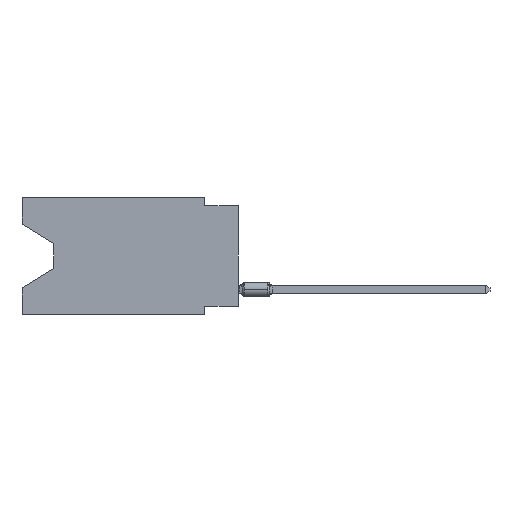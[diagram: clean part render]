
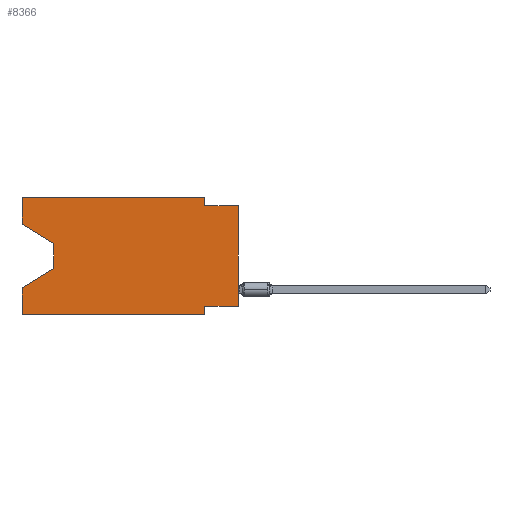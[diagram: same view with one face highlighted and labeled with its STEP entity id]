
A CAD part, left-side view. The second image highlights one B-rep face of the part: STEP entity #8366.
In plain terms, the highlighted planar face has unit normal (-1, 0, 0).
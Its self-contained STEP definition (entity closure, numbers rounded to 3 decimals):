
#251 = LINE ( 'NONE', #2073, #12682 ) ;
#1087 = VERTEX_POINT ( 'NONE', #7976 ) ;
#1093 = LINE ( 'NONE', #2813, #13261 ) ;
#1193 = DIRECTION ( 'NONE',  ( 0., -0.855, -0.519 ) ) ;
#1688 = LINE ( 'NONE', #13062, #12560 ) ;
#1826 = CARTESIAN_POINT ( 'NONE',  ( 0., 0., -0.635 ) ) ;
#1995 = EDGE_CURVE ( 'NONE', #4940, #10444, #19804, .T. ) ;
#2073 = CARTESIAN_POINT ( 'NONE',  ( 0., 16.383, 0. ) ) ;
#2531 = CARTESIAN_POINT ( 'NONE',  ( 0., 0., 0. ) ) ;
#2554 = EDGE_CURVE ( 'NONE', #6788, #12867, #10756, .T. ) ;
#2598 = CARTESIAN_POINT ( 'NONE',  ( 0., 16.383, -2.038 ) ) ;
#2666 = EDGE_CURVE ( 'NONE', #1087, #6656, #3111, .T. ) ;
#2712 = CARTESIAN_POINT ( 'NONE',  ( 0., 2.54, -0.635 ) ) ;
#2813 = CARTESIAN_POINT ( 'NONE',  ( 0., 16.383, 0. ) ) ;
#2944 = DIRECTION ( 'NONE',  ( 0., 0., -1. ) ) ;
#3111 = LINE ( 'NONE', #9673, #4296 ) ;
#3185 = CARTESIAN_POINT ( 'NONE',  ( 0., 16.383, -6.852 ) ) ;
#3435 = VECTOR ( 'NONE', #15576, 1000. ) ;
#3577 = ORIENTED_EDGE ( 'NONE', *, *, #8878, .F. ) ;
#4155 = LINE ( 'NONE', #7382, #7997 ) ;
#4232 = VECTOR ( 'NONE', #18378, 1000. ) ;
#4296 = VECTOR ( 'NONE', #14611, 1000. ) ;
#4940 = VERTEX_POINT ( 'NONE', #19956 ) ;
#5105 = ORIENTED_EDGE ( 'NONE', *, *, #1995, .T. ) ;
#5122 = CARTESIAN_POINT ( 'NONE',  ( 0., 16.383, -8.89 ) ) ;
#5468 = AXIS2_PLACEMENT_3D ( 'NONE', #16095, #17806, #19206 ) ;
#5704 = CARTESIAN_POINT ( 'NONE',  ( 0., 0., -0.635 ) ) ;
#6019 = FACE_OUTER_BOUND ( 'NONE', #6033, .T. ) ;
#6023 = LINE ( 'NONE', #5704, #3435 ) ;
#6033 = EDGE_LOOP ( 'NONE', ( #15017, #9505, #20596, #15298, #5105, #17332, #7921, #18885, #9639, #10597, #13761, #3577 ) ) ;
#6114 = LINE ( 'NONE', #9434, #14827 ) ;
#6656 = VERTEX_POINT ( 'NONE', #3185 ) ;
#6788 = VERTEX_POINT ( 'NONE', #15306 ) ;
#7232 = DIRECTION ( 'NONE',  ( 0., 0., 1. ) ) ;
#7358 = VERTEX_POINT ( 'NONE', #12612 ) ;
#7382 = CARTESIAN_POINT ( 'NONE',  ( 0., 13.97, -3.505 ) ) ;
#7545 = VECTOR ( 'NONE', #18416, 1000. ) ;
#7596 = EDGE_CURVE ( 'NONE', #7358, #9245, #8733, .T. ) ;
#7603 = VECTOR ( 'NONE', #2944, 1000. ) ;
#7921 = ORIENTED_EDGE ( 'NONE', *, *, #7596, .F. ) ;
#7976 = CARTESIAN_POINT ( 'NONE',  ( 0., 13.97, -5.385 ) ) ;
#7997 = VECTOR ( 'NONE', #10701, 1000. ) ;
#8366 = ADVANCED_FACE ( 'NONE', ( #6019 ), #10959, .F. ) ;
#8733 = LINE ( 'NONE', #13456, #4232 ) ;
#8878 = EDGE_CURVE ( 'NONE', #6788, #16752, #251, .T. ) ;
#9245 = VERTEX_POINT ( 'NONE', #19967 ) ;
#9284 = LINE ( 'NONE', #14424, #7603 ) ;
#9310 = CARTESIAN_POINT ( 'NONE',  ( 0., 13.97, -3.505 ) ) ;
#9429 = EDGE_CURVE ( 'NONE', #16518, #16681, #6023, .T. ) ;
#9434 = CARTESIAN_POINT ( 'NONE',  ( 0., 16.383, 0. ) ) ;
#9505 = ORIENTED_EDGE ( 'NONE', *, *, #15596, .T. ) ;
#9639 = ORIENTED_EDGE ( 'NONE', *, *, #9429, .F. ) ;
#9673 = CARTESIAN_POINT ( 'NONE',  ( 0., 13.97, -5.385 ) ) ;
#10304 = CARTESIAN_POINT ( 'NONE',  ( 0., 16.383, 0. ) ) ;
#10444 = VERTEX_POINT ( 'NONE', #14967 ) ;
#10597 = ORIENTED_EDGE ( 'NONE', *, *, #18918, .F. ) ;
#10701 = DIRECTION ( 'NONE',  ( 0., 0., -1. ) ) ;
#10756 = LINE ( 'NONE', #2598, #20204 ) ;
#10959 = PLANE ( 'NONE',  #5468 ) ;
#12098 = CARTESIAN_POINT ( 'NONE',  ( 0., 2.54, 0. ) ) ;
#12560 = VECTOR ( 'NONE', #16192, 1000. ) ;
#12612 = CARTESIAN_POINT ( 'NONE',  ( 0., 0., -8.255 ) ) ;
#12632 = VERTEX_POINT ( 'NONE', #12098 ) ;
#12682 = VECTOR ( 'NONE', #7232, 1000. ) ;
#12854 = DIRECTION ( 'NONE',  ( 0., -1., 0. ) ) ;
#12867 = VERTEX_POINT ( 'NONE', #9310 ) ;
#13062 = CARTESIAN_POINT ( 'NONE',  ( 0., 2.54, 0. ) ) ;
#13261 = VECTOR ( 'NONE', #20306, 1000. ) ;
#13391 = VECTOR ( 'NONE', #18939, 1000. ) ;
#13456 = CARTESIAN_POINT ( 'NONE',  ( 0., 0., -8.255 ) ) ;
#13761 = ORIENTED_EDGE ( 'NONE', *, *, #15255, .F. ) ;
#13795 = LINE ( 'NONE', #2531, #13391 ) ;
#14424 = CARTESIAN_POINT ( 'NONE',  ( 0., 2.54, -8.89 ) ) ;
#14611 = DIRECTION ( 'NONE',  ( 0., 0.855, -0.519 ) ) ;
#14827 = VECTOR ( 'NONE', #12854, 1000. ) ;
#14859 = EDGE_CURVE ( 'NONE', #9245, #10444, #9284, .T. ) ;
#14967 = CARTESIAN_POINT ( 'NONE',  ( 0., 2.54, -8.89 ) ) ;
#15017 = ORIENTED_EDGE ( 'NONE', *, *, #2554, .T. ) ;
#15255 = EDGE_CURVE ( 'NONE', #16752, #12632, #6114, .T. ) ;
#15298 = ORIENTED_EDGE ( 'NONE', *, *, #20014, .F. ) ;
#15306 = CARTESIAN_POINT ( 'NONE',  ( 0., 16.383, -2.038 ) ) ;
#15576 = DIRECTION ( 'NONE',  ( 0., -1., 0. ) ) ;
#15596 = EDGE_CURVE ( 'NONE', #12867, #1087, #4155, .T. ) ;
#16095 = CARTESIAN_POINT ( 'NONE',  ( 0., 16.383, 0. ) ) ;
#16192 = DIRECTION ( 'NONE',  ( 0., 0., -1. ) ) ;
#16518 = VERTEX_POINT ( 'NONE', #2712 ) ;
#16681 = VERTEX_POINT ( 'NONE', #1826 ) ;
#16752 = VERTEX_POINT ( 'NONE', #10304 ) ;
#17184 = EDGE_CURVE ( 'NONE', #7358, #16681, #13795, .T. ) ;
#17332 = ORIENTED_EDGE ( 'NONE', *, *, #14859, .F. ) ;
#17806 = DIRECTION ( 'NONE',  ( 1., 0., 0. ) ) ;
#18378 = DIRECTION ( 'NONE',  ( 0., 1., 0. ) ) ;
#18416 = DIRECTION ( 'NONE',  ( 0., -1., 0. ) ) ;
#18885 = ORIENTED_EDGE ( 'NONE', *, *, #17184, .T. ) ;
#18918 = EDGE_CURVE ( 'NONE', #12632, #16518, #1688, .T. ) ;
#18939 = DIRECTION ( 'NONE',  ( 0., 0., 1. ) ) ;
#19206 = DIRECTION ( 'NONE',  ( 0., 0., -1. ) ) ;
#19804 = LINE ( 'NONE', #5122, #7545 ) ;
#19956 = CARTESIAN_POINT ( 'NONE',  ( 0., 16.383, -8.89 ) ) ;
#19967 = CARTESIAN_POINT ( 'NONE',  ( 0., 2.54, -8.255 ) ) ;
#20014 = EDGE_CURVE ( 'NONE', #4940, #6656, #1093, .T. ) ;
#20204 = VECTOR ( 'NONE', #1193, 1000. ) ;
#20306 = DIRECTION ( 'NONE',  ( 0., 0., 1. ) ) ;
#20596 = ORIENTED_EDGE ( 'NONE', *, *, #2666, .T. ) ;
